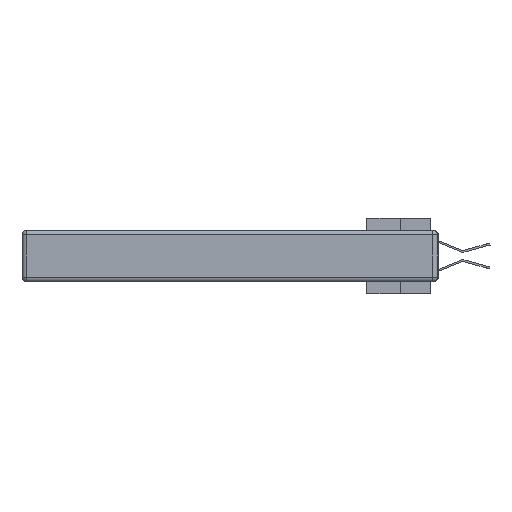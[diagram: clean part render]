
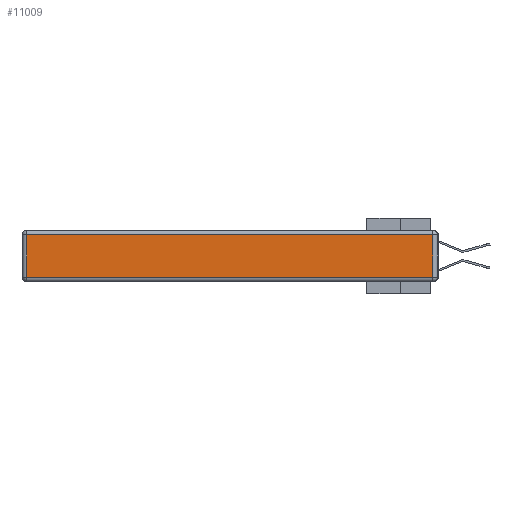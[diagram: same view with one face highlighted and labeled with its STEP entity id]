
A CAD part, left-side view. The second image highlights one B-rep face of the part: STEP entity #11009.
In plain terms, the highlighted planar face has unit normal (-1, 0, 0).
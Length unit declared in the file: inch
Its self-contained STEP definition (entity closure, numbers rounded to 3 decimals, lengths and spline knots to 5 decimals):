
#205 = VECTOR ( 'NONE', #8896, 39.37008 ) ;
#2399 = CARTESIAN_POINT ( 'NONE',  ( 0., 2.75, -0.03 ) ) ;
#3539 = VERTEX_POINT ( 'NONE', #26198 ) ;
#3763 = CARTESIAN_POINT ( 'NONE',  ( 0., 0.03, -0.313 ) ) ;
#4059 = DIRECTION ( 'NONE',  ( 0., 0., 1. ) ) ;
#4198 = VERTEX_POINT ( 'NONE', #3763 ) ;
#4905 = CARTESIAN_POINT ( 'NONE',  ( 0., 0.03, -0.03 ) ) ;
#6084 = VERTEX_POINT ( 'NONE', #4905 ) ;
#6481 = ORIENTED_EDGE ( 'NONE', *, *, #8149, .T. ) ;
#6691 = CARTESIAN_POINT ( 'NONE',  ( 0., 0., -0.343 ) ) ;
#6907 = EDGE_CURVE ( 'NONE', #4198, #6084, #27901, .T. ) ;
#7112 = DIRECTION ( 'NONE',  ( 0., 1., 0. ) ) ;
#7401 = DIRECTION ( 'NONE',  ( 0., -1., 0. ) ) ;
#8149 = EDGE_CURVE ( 'NONE', #6084, #3539, #8719, .T. ) ;
#8577 = CARTESIAN_POINT ( 'NONE',  ( 0., 0.03, -0.343 ) ) ;
#8719 = LINE ( 'NONE', #2399, #18878 ) ;
#8814 = VERTEX_POINT ( 'NONE', #30606 ) ;
#8896 = DIRECTION ( 'NONE',  ( 0., 0., -1. ) ) ;
#8998 = DIRECTION ( 'NONE',  ( -1., 0., 0. ) ) ;
#9127 = LINE ( 'NONE', #17285, #18908 ) ;
#11009 = ADVANCED_FACE ( 'NONE', ( #20191 ), #23501, .T. ) ;
#12004 = EDGE_LOOP ( 'NONE', ( #12369, #24536, #6481, #30331 ) ) ;
#12369 = ORIENTED_EDGE ( 'NONE', *, *, #13468, .T. ) ;
#13468 = EDGE_CURVE ( 'NONE', #8814, #4198, #9127, .T. ) ;
#13722 = LINE ( 'NONE', #21287, #205 ) ;
#16220 = DIRECTION ( 'NONE',  ( 0., 0., 1. ) ) ;
#17285 = CARTESIAN_POINT ( 'NONE',  ( 0., 0., -0.313 ) ) ;
#18650 = EDGE_CURVE ( 'NONE', #3539, #8814, #13722, .T. ) ;
#18878 = VECTOR ( 'NONE', #7112, 39.37008 ) ;
#18908 = VECTOR ( 'NONE', #7401, 39.37008 ) ;
#20191 = FACE_OUTER_BOUND ( 'NONE', #12004, .T. ) ;
#20415 = VECTOR ( 'NONE', #4059, 39.37008 ) ;
#21287 = CARTESIAN_POINT ( 'NONE',  ( 0., 2.72, -0.343 ) ) ;
#23501 = PLANE ( 'NONE',  #23831 ) ;
#23831 = AXIS2_PLACEMENT_3D ( 'NONE', #6691, #8998, #16220 ) ;
#24536 = ORIENTED_EDGE ( 'NONE', *, *, #6907, .T. ) ;
#26198 = CARTESIAN_POINT ( 'NONE',  ( 0., 2.72, -0.03 ) ) ;
#27901 = LINE ( 'NONE', #8577, #20415 ) ;
#30331 = ORIENTED_EDGE ( 'NONE', *, *, #18650, .T. ) ;
#30606 = CARTESIAN_POINT ( 'NONE',  ( 0., 2.72, -0.313 ) ) ;
